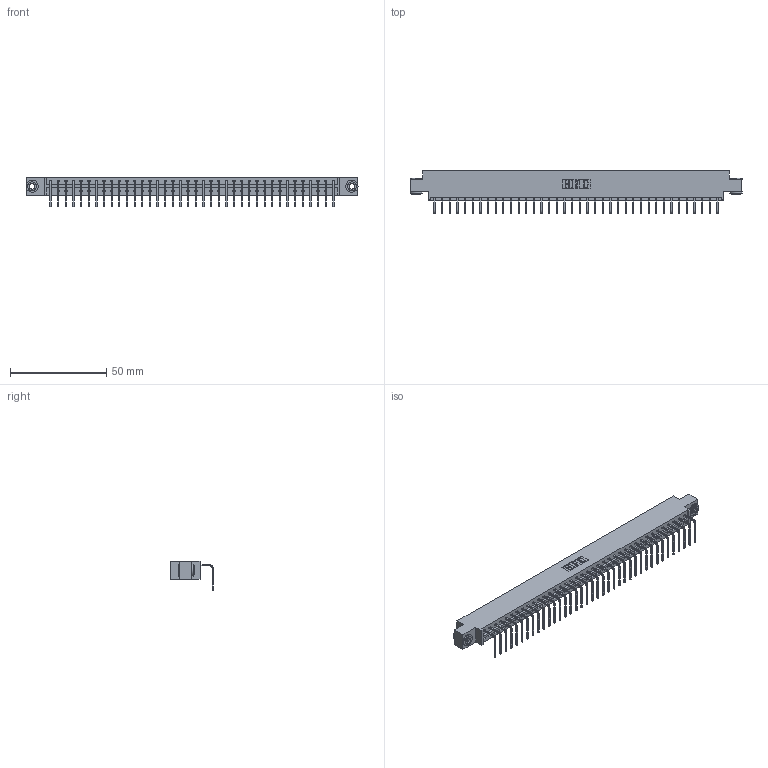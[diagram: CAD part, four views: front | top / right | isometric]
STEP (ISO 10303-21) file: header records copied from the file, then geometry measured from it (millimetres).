
FILE_DESCRIPTION (( 'STEP AP203' ), '1' );
FILE_NAME ('333-038-558-603.STEP', '2018-08-03T12:05:07', ( '' ), ( '' ), 'SwSTEP 2.0', 'SolidWorks 2016', '' );
FILE_SCHEMA (( 'CONFIG_CONTROL_DESIGN' ));
Length unit declared in the file: inch
Products named in the file (4): 345-292-001_558 Tail - 2; 345-250-002_345-250-002-102; 333-038-558-603; 333 Part_Offset - .156 Dia - TH
Assembly tree (41 placements, depth 2):
  333-038-558-603
    333 Part_Offset - .156 Dia - TH
    345-292-001_558 Tail - 2  x38
    345-250-002_345-250-002-102  x2
Bounding box: 172.11 x 22.17 x 15.37 mm (x, y, z)
Volume: 17203 mm3; surface area: 19789.1 mm2
Topology: 41 solids, 41 shells, 2436 faces, 7315 edges, 4822 vertices
Faces by surface type: plane 1756, cylinder 672, cone 8
Entity records: 24614 total; most frequent: CARTESIAN_POINT 4227, ORIENTED_EDGE 4194, DIRECTION 3607, EDGE_CURVE 2097, LINE 1945, VECTOR 1945, VERTEX_POINT 1394, AXIS2_PLACEMENT_3D 831
